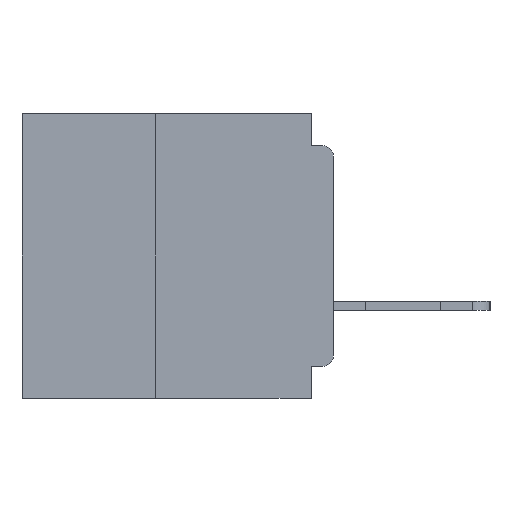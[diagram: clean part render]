
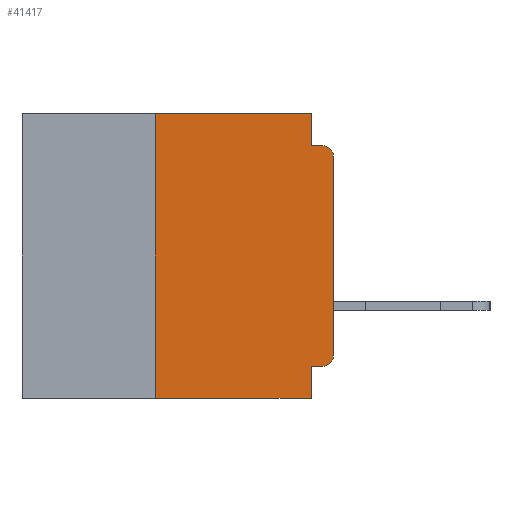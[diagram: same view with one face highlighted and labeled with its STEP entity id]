
A CAD part, left-side view. The second image highlights one B-rep face of the part: STEP entity #41417.
In plain terms, the highlighted planar face has unit normal (-1, 0, 0).
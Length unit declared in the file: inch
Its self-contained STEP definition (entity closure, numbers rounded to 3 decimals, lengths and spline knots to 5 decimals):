
#270 = ORIENTED_EDGE ( 'NONE', *, *, #37518, .F. ) ;
#757 = CIRCLE ( 'NONE', #42606, 0.015 ) ;
#1359 = CARTESIAN_POINT ( 'NONE',  ( 0., 0., 0. ) ) ;
#2219 = VECTOR ( 'NONE', #23431, 39.37008 ) ;
#2298 = CARTESIAN_POINT ( 'NONE',  ( 0., 0.031, -0.4 ) ) ;
#2348 = DIRECTION ( 'NONE',  ( 0., 0., -1. ) ) ;
#2912 = DIRECTION ( 'NONE',  ( 0., -1., 0. ) ) ;
#3357 = ORIENTED_EDGE ( 'NONE', *, *, #20473, .T. ) ;
#4061 = ORIENTED_EDGE ( 'NONE', *, *, #18182, .T. ) ;
#4286 = EDGE_LOOP ( 'NONE', ( #27255, #4061, #21557, #24669, #36073, #28350, #30140, #40835, #270, #3357 ) ) ;
#5017 = AXIS2_PLACEMENT_3D ( 'NONE', #39058, #19408, #42359 ) ;
#5201 = CARTESIAN_POINT ( 'NONE',  ( 0., 0.031, -0.045 ) ) ;
#5304 = DIRECTION ( 'NONE',  ( 0., -1., 0. ) ) ;
#5546 = EDGE_CURVE ( 'NONE', #13856, #38562, #11001, .T. ) ;
#6553 = CARTESIAN_POINT ( 'NONE',  ( 0., 0., -0.045 ) ) ;
#6581 = EDGE_CURVE ( 'NONE', #36708, #10749, #28885, .T. ) ;
#9034 = EDGE_CURVE ( 'NONE', #23269, #10209, #31044, .T. ) ;
#10209 = VERTEX_POINT ( 'NONE', #11330 ) ;
#10749 = VERTEX_POINT ( 'NONE', #30530 ) ;
#10911 = DIRECTION ( 'NONE',  ( 0., 0., -1. ) ) ;
#11001 = LINE ( 'NONE', #23901, #2219 ) ;
#11330 = CARTESIAN_POINT ( 'NONE',  ( 0., 0., -0.06 ) ) ;
#12101 = CARTESIAN_POINT ( 'NONE',  ( 0., 0., -0.355 ) ) ;
#12274 = VERTEX_POINT ( 'NONE', #42093 ) ;
#12317 = LINE ( 'NONE', #34787, #30834 ) ;
#12700 = VERTEX_POINT ( 'NONE', #17436 ) ;
#13759 = LINE ( 'NONE', #22932, #22453 ) ;
#13856 = VERTEX_POINT ( 'NONE', #33146 ) ;
#14087 = CARTESIAN_POINT ( 'NONE',  ( 0., 0.437, 0. ) ) ;
#14113 = LINE ( 'NONE', #6553, #39233 ) ;
#15537 = EDGE_CURVE ( 'NONE', #18522, #13856, #30827, .T. ) ;
#15579 = LINE ( 'NONE', #12101, #32044 ) ;
#16765 = VERTEX_POINT ( 'NONE', #41863 ) ;
#16776 = CARTESIAN_POINT ( 'NONE',  ( 0., 0.015, -0.06 ) ) ;
#17436 = CARTESIAN_POINT ( 'NONE',  ( 0., 0.015, -0.045 ) ) ;
#18182 = EDGE_CURVE ( 'NONE', #10209, #12700, #757, .T. ) ;
#18427 = CARTESIAN_POINT ( 'NONE',  ( 0., 0.25, 0. ) ) ;
#18522 = VERTEX_POINT ( 'NONE', #18427 ) ;
#18667 = CIRCLE ( 'NONE', #5017, 0.015 ) ;
#19408 = DIRECTION ( 'NONE',  ( -1., 0., 0. ) ) ;
#20026 = DIRECTION ( 'NONE',  ( 0., 0., -1. ) ) ;
#20121 = VECTOR ( 'NONE', #2348, 39.37008 ) ;
#20473 = EDGE_CURVE ( 'NONE', #12274, #23269, #18667, .T. ) ;
#21222 = VECTOR ( 'NONE', #34311, 39.37008 ) ;
#21557 = ORIENTED_EDGE ( 'NONE', *, *, #32057, .F. ) ;
#22453 = VECTOR ( 'NONE', #32864, 39.37008 ) ;
#22776 = EDGE_CURVE ( 'NONE', #16765, #10749, #12317, .T. ) ;
#22932 = CARTESIAN_POINT ( 'NONE',  ( 0., 0.25, -0.4 ) ) ;
#23269 = VERTEX_POINT ( 'NONE', #40578 ) ;
#23431 = DIRECTION ( 'NONE',  ( 0., 0., -1. ) ) ;
#23901 = CARTESIAN_POINT ( 'NONE',  ( 0., 0.031, 0. ) ) ;
#24066 = CARTESIAN_POINT ( 'NONE',  ( 0., 0.031, -0.355 ) ) ;
#24669 = ORIENTED_EDGE ( 'NONE', *, *, #5546, .F. ) ;
#27255 = ORIENTED_EDGE ( 'NONE', *, *, #9034, .T. ) ;
#27301 = PLANE ( 'NONE',  #36693 ) ;
#28350 = ORIENTED_EDGE ( 'NONE', *, *, #36480, .F. ) ;
#28885 = LINE ( 'NONE', #2298, #20121 ) ;
#29263 = CARTESIAN_POINT ( 'NONE',  ( 0., 0.437, 0. ) ) ;
#29624 = FACE_OUTER_BOUND ( 'NONE', #4286, .T. ) ;
#30140 = ORIENTED_EDGE ( 'NONE', *, *, #22776, .T. ) ;
#30530 = CARTESIAN_POINT ( 'NONE',  ( 0., 0.031, -0.4 ) ) ;
#30618 = DIRECTION ( 'NONE',  ( 1., 0., 0. ) ) ;
#30827 = LINE ( 'NONE', #29263, #39482 ) ;
#30834 = VECTOR ( 'NONE', #5304, 39.37008 ) ;
#31044 = LINE ( 'NONE', #1359, #21222 ) ;
#31785 = DIRECTION ( 'NONE',  ( 0., 1., 0. ) ) ;
#32044 = VECTOR ( 'NONE', #31785, 39.37008 ) ;
#32057 = EDGE_CURVE ( 'NONE', #38562, #12700, #14113, .T. ) ;
#32864 = DIRECTION ( 'NONE',  ( 0., 0., 1. ) ) ;
#33146 = CARTESIAN_POINT ( 'NONE',  ( 0., 0.031, 0. ) ) ;
#34311 = DIRECTION ( 'NONE',  ( 0., 0., 1. ) ) ;
#34787 = CARTESIAN_POINT ( 'NONE',  ( 0., 0.437, -0.4 ) ) ;
#36073 = ORIENTED_EDGE ( 'NONE', *, *, #15537, .F. ) ;
#36480 = EDGE_CURVE ( 'NONE', #16765, #18522, #13759, .T. ) ;
#36693 = AXIS2_PLACEMENT_3D ( 'NONE', #14087, #30618, #10911 ) ;
#36708 = VERTEX_POINT ( 'NONE', #24066 ) ;
#37518 = EDGE_CURVE ( 'NONE', #12274, #36708, #15579, .T. ) ;
#38562 = VERTEX_POINT ( 'NONE', #5201 ) ;
#39058 = CARTESIAN_POINT ( 'NONE',  ( 0., 0.015, -0.34 ) ) ;
#39233 = VECTOR ( 'NONE', #39287, 39.37008 ) ;
#39287 = DIRECTION ( 'NONE',  ( 0., -1., 0. ) ) ;
#39482 = VECTOR ( 'NONE', #2912, 39.37008 ) ;
#39666 = DIRECTION ( 'NONE',  ( -1., 0., 0. ) ) ;
#40578 = CARTESIAN_POINT ( 'NONE',  ( 0., 0., -0.34 ) ) ;
#40835 = ORIENTED_EDGE ( 'NONE', *, *, #6581, .F. ) ;
#41417 = ADVANCED_FACE ( 'NONE', ( #29624 ), #27301, .F. ) ;
#41863 = CARTESIAN_POINT ( 'NONE',  ( 0., 0.25, -0.4 ) ) ;
#42093 = CARTESIAN_POINT ( 'NONE',  ( 0., 0.015, -0.355 ) ) ;
#42359 = DIRECTION ( 'NONE',  ( 0., 0., -1. ) ) ;
#42606 = AXIS2_PLACEMENT_3D ( 'NONE', #16776, #39666, #20026 ) ;
